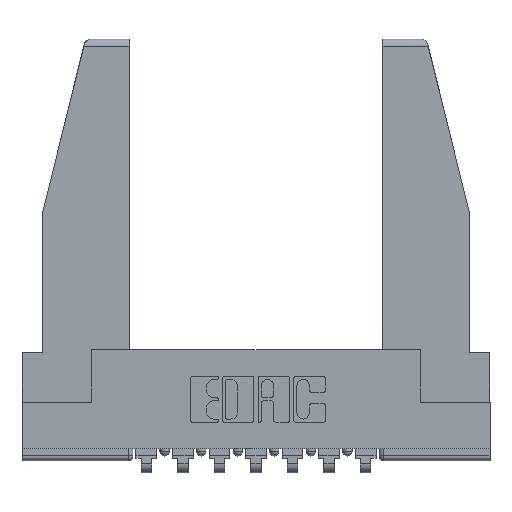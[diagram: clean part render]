
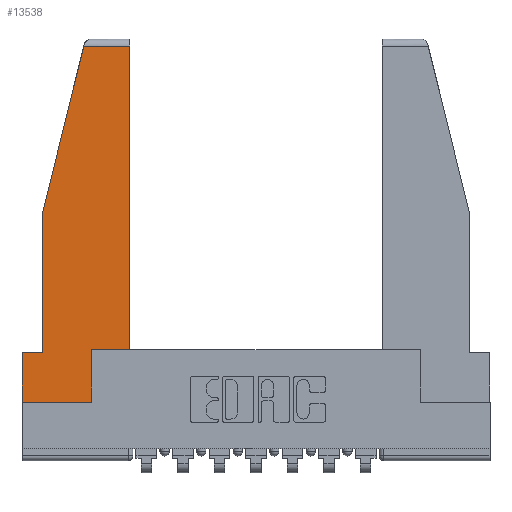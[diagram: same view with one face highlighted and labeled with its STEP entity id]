
A CAD part, top view. The second image highlights one B-rep face of the part: STEP entity #13538.
In plain terms, the highlighted planar face has unit normal (0, 0, 1).
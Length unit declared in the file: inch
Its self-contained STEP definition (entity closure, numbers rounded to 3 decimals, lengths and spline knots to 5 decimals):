
#17 = CARTESIAN_POINT ( 'NONE',  ( 0., 0., 0. ) ) ;
#120 = AXIS2_PLACEMENT_3D ( 'NONE', #17, #4251, #8258 ) ;
#275 = VERTEX_POINT ( 'NONE', #3930 ) ;
#367 = CARTESIAN_POINT ( 'NONE',  ( 0.271, 1.55, 0. ) ) ;
#450 = VECTOR ( 'NONE', #2339, 39.37008 ) ;
#628 = VERTEX_POINT ( 'NONE', #10853 ) ;
#631 = EDGE_CURVE ( 'NONE', #6824, #11566, #1673, .T. ) ;
#652 = ORIENTED_EDGE ( 'NONE', *, *, #631, .T. ) ;
#710 = DIRECTION ( 'NONE',  ( -1., 0., 0. ) ) ;
#899 = PLANE ( 'NONE',  #120 ) ;
#944 = VECTOR ( 'NONE', #5774, 39.37008 ) ;
#964 = VERTEX_POINT ( 'NONE', #5831 ) ;
#971 = LINE ( 'NONE', #4246, #5600 ) ;
#1038 = FACE_OUTER_BOUND ( 'NONE', #1784, .T. ) ;
#1257 = LINE ( 'NONE', #367, #7163 ) ;
#1508 = EDGE_CURVE ( 'NONE', #628, #275, #2405, .T. ) ;
#1673 = LINE ( 'NONE', #10091, #944 ) ;
#1784 = EDGE_LOOP ( 'NONE', ( #6759, #2520, #12215, #6906, #3287, #9038, #652, #13552, #5024 ) ) ;
#2339 = DIRECTION ( 'NONE',  ( 0., -1., 0. ) ) ;
#2405 = LINE ( 'NONE', #7857, #450 ) ;
#2456 = DIRECTION ( 'NONE',  ( -0.239, -0.971, 0. ) ) ;
#2480 = CARTESIAN_POINT ( 'NONE',  ( 0., 0., 0. ) ) ;
#2520 = ORIENTED_EDGE ( 'NONE', *, *, #8777, .T. ) ;
#2658 = DIRECTION ( 'NONE',  ( 0., 1., 0. ) ) ;
#2889 = CARTESIAN_POINT ( 'NONE',  ( 0., 1.52, 0. ) ) ;
#2971 = VECTOR ( 'NONE', #5212, 39.37008 ) ;
#3031 = CARTESIAN_POINT ( 'NONE',  ( 0.297, 0., 0. ) ) ;
#3132 = DIRECTION ( 'NONE',  ( -1., 0., 0. ) ) ;
#3287 = ORIENTED_EDGE ( 'NONE', *, *, #10721, .T. ) ;
#3455 = VECTOR ( 'NONE', #710, 39.37008 ) ;
#3864 = CARTESIAN_POINT ( 'NONE',  ( 0., 0.21, 0. ) ) ;
#3930 = CARTESIAN_POINT ( 'NONE',  ( 0.086, 0.21, 0. ) ) ;
#4059 = VERTEX_POINT ( 'NONE', #10698 ) ;
#4144 = VECTOR ( 'NONE', #2658, 39.37008 ) ;
#4246 = CARTESIAN_POINT ( 'NONE',  ( 0., 0.21, 0. ) ) ;
#4251 = DIRECTION ( 'NONE',  ( 0., 0., 1. ) ) ;
#4625 = CARTESIAN_POINT ( 'NONE',  ( 0.297, 0.223, 0. ) ) ;
#5024 = ORIENTED_EDGE ( 'NONE', *, *, #7263, .T. ) ;
#5195 = VECTOR ( 'NONE', #5721, 39.37008 ) ;
#5212 = DIRECTION ( 'NONE',  ( 0., 1., 0. ) ) ;
#5215 = VECTOR ( 'NONE', #9841, 39.37008 ) ;
#5600 = VECTOR ( 'NONE', #3132, 39.37008 ) ;
#5721 = DIRECTION ( 'NONE',  ( 0., -1., 0. ) ) ;
#5774 = DIRECTION ( 'NONE',  ( 1., 0., 0. ) ) ;
#5831 = CARTESIAN_POINT ( 'NONE',  ( 0.297, 0.223, 0. ) ) ;
#6312 = LINE ( 'NONE', #6373, #2971 ) ;
#6373 = CARTESIAN_POINT ( 'NONE',  ( 0.297, 0., 0. ) ) ;
#6652 = EDGE_CURVE ( 'NONE', #11566, #964, #6312, .T. ) ;
#6759 = ORIENTED_EDGE ( 'NONE', *, *, #9249, .T. ) ;
#6824 = VERTEX_POINT ( 'NONE', #2480 ) ;
#6906 = ORIENTED_EDGE ( 'NONE', *, *, #1508, .T. ) ;
#7163 = VECTOR ( 'NONE', #2456, 39.37008 ) ;
#7246 = VERTEX_POINT ( 'NONE', #10597 ) ;
#7263 = EDGE_CURVE ( 'NONE', #964, #7647, #10867, .T. ) ;
#7566 = LINE ( 'NONE', #8799, #5195 ) ;
#7647 = VERTEX_POINT ( 'NONE', #12521 ) ;
#7857 = CARTESIAN_POINT ( 'NONE',  ( 0.086, 0.8, 0. ) ) ;
#8258 = DIRECTION ( 'NONE',  ( 1., 0., 0. ) ) ;
#8777 = EDGE_CURVE ( 'NONE', #7246, #4059, #12173, .T. ) ;
#8799 = CARTESIAN_POINT ( 'NONE',  ( 0., 0.21, 0. ) ) ;
#9038 = ORIENTED_EDGE ( 'NONE', *, *, #11788, .T. ) ;
#9249 = EDGE_CURVE ( 'NONE', #7647, #7246, #12086, .T. ) ;
#9841 = DIRECTION ( 'NONE',  ( 1., 0., 0. ) ) ;
#10091 = CARTESIAN_POINT ( 'NONE',  ( 0., 0., 0. ) ) ;
#10282 = VERTEX_POINT ( 'NONE', #3864 ) ;
#10597 = CARTESIAN_POINT ( 'NONE',  ( 0.461, 1.52, 0. ) ) ;
#10698 = CARTESIAN_POINT ( 'NONE',  ( 0.2636, 1.52, 0. ) ) ;
#10721 = EDGE_CURVE ( 'NONE', #275, #10282, #971, .T. ) ;
#10853 = CARTESIAN_POINT ( 'NONE',  ( 0.086, 0.8, 0. ) ) ;
#10867 = LINE ( 'NONE', #4625, #5215 ) ;
#11123 = CARTESIAN_POINT ( 'NONE',  ( 0.461, 0.223, 0. ) ) ;
#11566 = VERTEX_POINT ( 'NONE', #3031 ) ;
#11770 = EDGE_CURVE ( 'NONE', #4059, #628, #1257, .T. ) ;
#11788 = EDGE_CURVE ( 'NONE', #10282, #6824, #7566, .T. ) ;
#12086 = LINE ( 'NONE', #11123, #4144 ) ;
#12173 = LINE ( 'NONE', #2889, #3455 ) ;
#12215 = ORIENTED_EDGE ( 'NONE', *, *, #11770, .T. ) ;
#12521 = CARTESIAN_POINT ( 'NONE',  ( 0.461, 0.223, 0. ) ) ;
#13538 = ADVANCED_FACE ( 'NONE', ( #1038 ), #899, .T. ) ;
#13552 = ORIENTED_EDGE ( 'NONE', *, *, #6652, .T. ) ;
